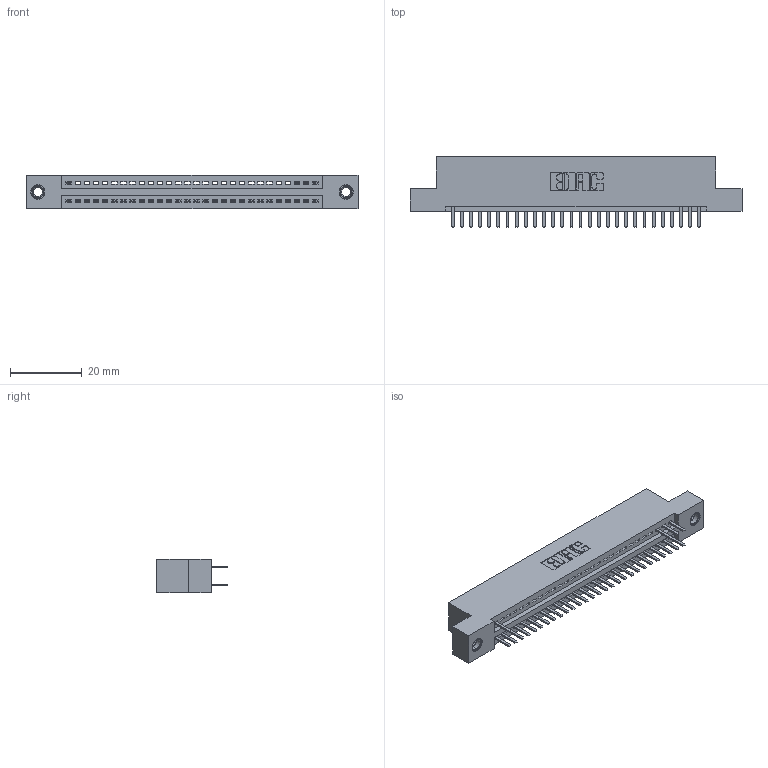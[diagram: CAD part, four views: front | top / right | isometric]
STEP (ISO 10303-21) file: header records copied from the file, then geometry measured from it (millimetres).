
FILE_DESCRIPTION (( 'STEP AP203' ), '1' );
FILE_NAME ('345-056-520-207.STEP', '2018-09-24T06:55:13', ( '' ), ( '' ), 'SwSTEP 2.0', 'SolidWorks 2016', '' );
FILE_SCHEMA (( 'CONFIG_CONTROL_DESIGN' ));
Length unit declared in the file: inch
Products named in the file (4): 345-292-001_345-293-120; 345-250-001_345-250-005-103; 345-056-520-207; 345 Part_Flush Mounting Lugs - 0.156 Dia-TI
Assembly tree (35 placements, depth 2):
  345-056-520-207
    345 Part_Flush Mounting Lugs - 0.156 Dia-TI
    345-292-001_345-293-120  x32
    345-250-001_345-250-005-103  x2
Bounding box: 92.33 x 19.68 x 9.4 mm (x, y, z)
Volume: 8595.1 mm3; surface area: 11206.4 mm2
Topology: 35 solids, 35 shells, 2106 faces, 6149 edges, 4006 vertices
Faces by surface type: plane 1400, cylinder 690, cone 12, torus 4
Entity records: 24386 total; most frequent: CARTESIAN_POINT 4199, ORIENTED_EDGE 4138, DIRECTION 3707, EDGE_CURVE 2069, VECTOR 1801, LINE 1801, VERTEX_POINT 1372, AXIS2_PLACEMENT_3D 953
